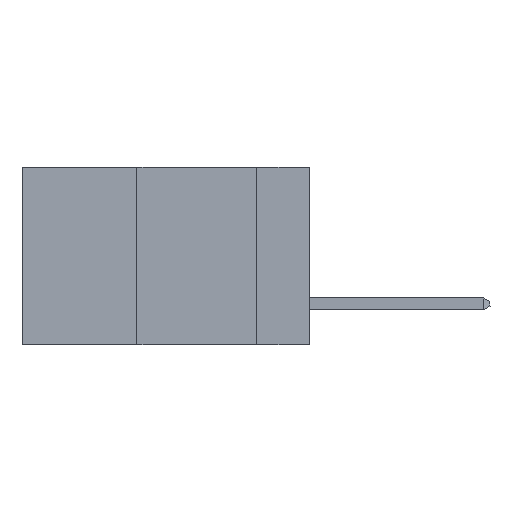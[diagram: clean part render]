
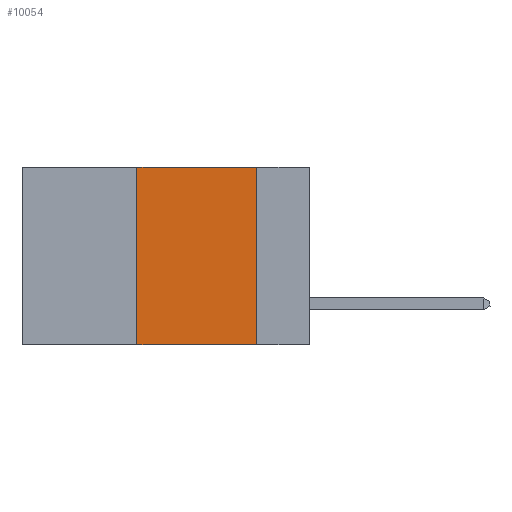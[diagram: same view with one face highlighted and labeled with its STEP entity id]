
A CAD part, left-side view. The second image highlights one B-rep face of the part: STEP entity #10054.
In plain terms, the highlighted planar face has unit normal (-1, 0, 0).
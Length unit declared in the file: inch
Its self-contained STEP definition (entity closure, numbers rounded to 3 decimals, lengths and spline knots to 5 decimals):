
#827 = VECTOR ( 'NONE', #4014, 39.37008 ) ;
#1258 = DIRECTION ( 'NONE',  ( 0., 0., 1. ) ) ;
#1280 = PLANE ( 'NONE',  #10086 ) ;
#1462 = DIRECTION ( 'NONE',  ( 0., 0., -1. ) ) ;
#1740 = EDGE_CURVE ( 'NONE', #5666, #4801, #8991, .T. ) ;
#2356 = ORIENTED_EDGE ( 'NONE', *, *, #6673, .F. ) ;
#2507 = LINE ( 'NONE', #8911, #9463 ) ;
#3158 = EDGE_CURVE ( 'NONE', #4801, #6092, #2507, .T. ) ;
#3165 = CARTESIAN_POINT ( 'NONE',  ( 0., 0.11, 0. ) ) ;
#3629 = CARTESIAN_POINT ( 'NONE',  ( 0., 0.36, 0. ) ) ;
#3991 = DIRECTION ( 'NONE',  ( 1., 0., 0. ) ) ;
#4014 = DIRECTION ( 'NONE',  ( 0., 0., -1. ) ) ;
#4747 = CARTESIAN_POINT ( 'NONE',  ( 0., 0.36, -0.37 ) ) ;
#4801 = VERTEX_POINT ( 'NONE', #7769 ) ;
#5129 = LINE ( 'NONE', #3165, #827 ) ;
#5141 = VECTOR ( 'NONE', #8111, 39.37008 ) ;
#5146 = EDGE_LOOP ( 'NONE', ( #2356, #9435, #9810, #9909 ) ) ;
#5658 = CARTESIAN_POINT ( 'NONE',  ( 0., 0.6, -0.37 ) ) ;
#5666 = VERTEX_POINT ( 'NONE', #4747 ) ;
#6092 = VERTEX_POINT ( 'NONE', #8704 ) ;
#6298 = EDGE_CURVE ( 'NONE', #5666, #7244, #8188, .T. ) ;
#6523 = DIRECTION ( 'NONE',  ( 0., -1., 0. ) ) ;
#6673 = EDGE_CURVE ( 'NONE', #6092, #7244, #5129, .T. ) ;
#7043 = VECTOR ( 'NONE', #1258, 39.37008 ) ;
#7244 = VERTEX_POINT ( 'NONE', #9458 ) ;
#7769 = CARTESIAN_POINT ( 'NONE',  ( 0., 0.36, 0. ) ) ;
#8111 = DIRECTION ( 'NONE',  ( 0., -1., 0. ) ) ;
#8150 = CARTESIAN_POINT ( 'NONE',  ( 0., 0.6, 0. ) ) ;
#8188 = LINE ( 'NONE', #5658, #5141 ) ;
#8704 = CARTESIAN_POINT ( 'NONE',  ( 0., 0.11, 0. ) ) ;
#8911 = CARTESIAN_POINT ( 'NONE',  ( 0., 0.6, 0. ) ) ;
#8991 = LINE ( 'NONE', #3629, #7043 ) ;
#9435 = ORIENTED_EDGE ( 'NONE', *, *, #3158, .F. ) ;
#9458 = CARTESIAN_POINT ( 'NONE',  ( 0., 0.11, -0.37 ) ) ;
#9463 = VECTOR ( 'NONE', #6523, 39.37008 ) ;
#9797 = FACE_OUTER_BOUND ( 'NONE', #5146, .T. ) ;
#9810 = ORIENTED_EDGE ( 'NONE', *, *, #1740, .F. ) ;
#9909 = ORIENTED_EDGE ( 'NONE', *, *, #6298, .T. ) ;
#10054 = ADVANCED_FACE ( 'NONE', ( #9797 ), #1280, .F. ) ;
#10086 = AXIS2_PLACEMENT_3D ( 'NONE', #8150, #3991, #1462 ) ;
